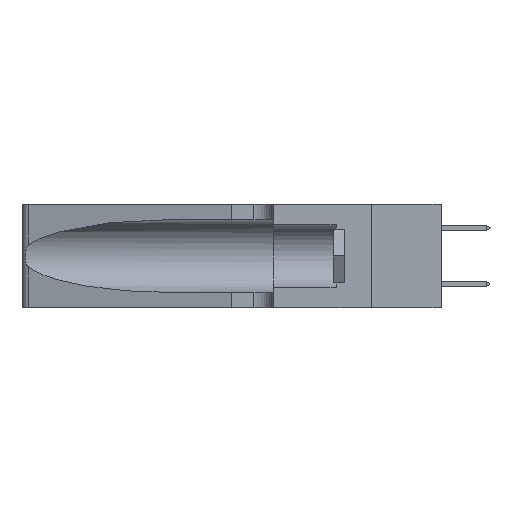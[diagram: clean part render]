
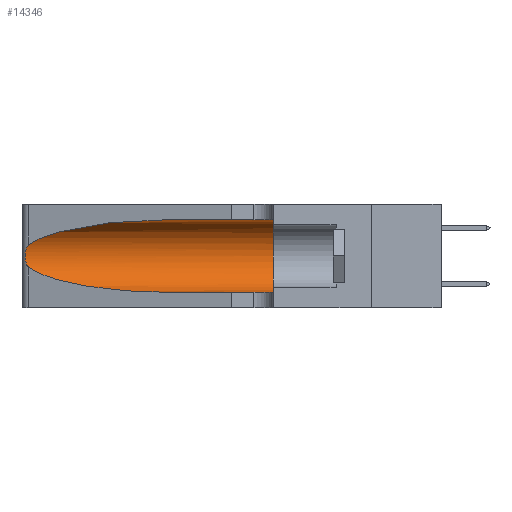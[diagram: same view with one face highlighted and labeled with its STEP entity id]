
A CAD part, left-side view. The second image highlights one B-rep face of the part: STEP entity #14346.
In plain terms, the highlighted cylindrical face has radius 3.308 mm (diameter 6.617 mm), a partial arc.
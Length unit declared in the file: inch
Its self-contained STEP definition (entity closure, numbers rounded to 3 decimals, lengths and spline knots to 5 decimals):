
#706 = DIRECTION ( 'NONE',  ( 0., -1., 0. ) ) ;
#932 = VERTEX_POINT ( 'NONE', #3091 ) ;
#1128 = CARTESIAN_POINT ( 'NONE',  ( 0.2373, 1.15595, 0.28018 ) ) ;
#1200 = CARTESIAN_POINT ( 'NONE',  ( 0.25487, 1.22718, 0.22369 ) ) ;
#1931 = VERTEX_POINT ( 'NONE', #32887 ) ;
#2377 = CARTESIAN_POINT ( 'NONE',  ( 0.2373, 1.15595, 0.08982 ) ) ;
#2533 = CARTESIAN_POINT ( 'NONE',  ( 0.26075, 1.23896, 0.19203 ) ) ;
#2657 = EDGE_CURVE ( 'NONE', #2901, #16434, #25597, .T. ) ;
#2893 = EDGE_CURVE ( 'NONE', #16434, #1931, #18274, .T. ) ;
#2901 = VERTEX_POINT ( 'NONE', #37509 ) ;
#3091 = CARTESIAN_POINT ( 'NONE',  ( 0.1305, 0.72297, 0.05475 ) ) ;
#3627 = ORIENTED_EDGE ( 'NONE', *, *, #18187, .F. ) ;
#3734 = AXIS2_PLACEMENT_3D ( 'NONE', #3744, #25972, #6998 ) ;
#3744 = CARTESIAN_POINT ( 'NONE',  ( 0.1305, 0.35, 0.185 ) ) ;
#4104 = ORIENTED_EDGE ( 'NONE', *, *, #6534, .F. ) ;
#4507 = CARTESIAN_POINT ( 'NONE',  ( 0.18966, 0.96281, 0.31525 ) ) ;
#4724 =( BOUNDED_CURVE ( )  B_SPLINE_CURVE ( 3, ( #40383, #2377, #24632, #5607 ),
 .UNSPECIFIED., .F., .F. ) 
 B_SPLINE_CURVE_WITH_KNOTS ( ( 4, 4 ),
 ( 3.44316, 4.71239 ),
 .UNSPECIFIED. ) 
 CURVE ( )  GEOMETRIC_REPRESENTATION_ITEM ( )  RATIONAL_B_SPLINE_CURVE ( ( 1., 0.87, 0.87, 1. ) ) 
 REPRESENTATION_ITEM ( '' )  );
#5063 = CARTESIAN_POINT ( 'NONE',  ( 0.1305, 0.35, 0.31525 ) ) ;
#5595 = DIRECTION ( 'NONE',  ( 0., -1., 0. ) ) ;
#5607 = CARTESIAN_POINT ( 'NONE',  ( 0.1305, 0.72297, 0.05475 ) ) ;
#5761 = CARTESIAN_POINT ( 'NONE',  ( 0.26017, 1.23833, 0.17102 ) ) ;
#6534 = EDGE_CURVE ( 'NONE', #2901, #16122, #35274, .T. ) ;
#6998 = DIRECTION ( 'NONE',  ( 0., 0., 1. ) ) ;
#8979 = CARTESIAN_POINT ( 'NONE',  ( 0.25789, 1.23486, 0.15765 ) ) ;
#9538 = DIRECTION ( 'NONE',  ( 0., 0., -1. ) ) ;
#10998 = CARTESIAN_POINT ( 'NONE',  ( 0.25487, 1.22718, 0.22369 ) ) ;
#12193 = CARTESIAN_POINT ( 'NONE',  ( 0.25555, 1.22993, 0.14849 ) ) ;
#12730 = CIRCLE ( 'NONE', #3734, 0.13025 ) ;
#14346 = ADVANCED_FACE ( 'NONE', ( #20648 ), #33510, .F. ) ;
#16107 = ORIENTED_EDGE ( 'NONE', *, *, #30903, .T. ) ;
#16122 = VERTEX_POINT ( 'NONE', #5063 ) ;
#16434 = VERTEX_POINT ( 'NONE', #1200 ) ;
#18187 = EDGE_CURVE ( 'NONE', #16122, #24683, #12730, .T. ) ;
#18274 = B_SPLINE_CURVE_WITH_KNOTS ( 'NONE', 3,
 ( #18295, #31002, #37370, #18429, #40533, #21575, #2533, #24783, #5761, #27948, #8979, #31133, #12193, #34324 ),
 .UNSPECIFIED., .F., .F.,
 ( 4, 2, 2, 2, 2, 2, 4 ),
 ( 0., 0.00027, 0.00053, 0.00107, 0.0016, 0.00187, 0.00214 ),
 .UNSPECIFIED. ) ;
#18295 = CARTESIAN_POINT ( 'NONE',  ( 0.25487, 1.22718, 0.22369 ) ) ;
#18429 = CARTESIAN_POINT ( 'NONE',  ( 0.25787, 1.23484, 0.2124 ) ) ;
#20053 = EDGE_CURVE ( 'NONE', #932, #24683, #27425, .T. ) ;
#20648 = FACE_OUTER_BOUND ( 'NONE', #21431, .T. ) ;
#21379 = ORIENTED_EDGE ( 'NONE', *, *, #2657, .T. ) ;
#21431 = EDGE_LOOP ( 'NONE', ( #21379, #26727, #16107, #35734, #3627, #4104 ) ) ;
#21575 = CARTESIAN_POINT ( 'NONE',  ( 0.26018, 1.23835, 0.19895 ) ) ;
#22123 = CARTESIAN_POINT ( 'NONE',  ( 0.1305, 1.61858, 0.185 ) ) ;
#24632 = CARTESIAN_POINT ( 'NONE',  ( 0.18966, 0.96281, 0.05475 ) ) ;
#24683 = VERTEX_POINT ( 'NONE', #31760 ) ;
#24783 = CARTESIAN_POINT ( 'NONE',  ( 0.26075, 1.23896, 0.178 ) ) ;
#25597 =( BOUNDED_CURVE ( )  B_SPLINE_CURVE ( 3, ( #29935, #4507, #1128, #10998 ),
 .UNSPECIFIED., .F., .F. ) 
 B_SPLINE_CURVE_WITH_KNOTS ( ( 4, 4 ),
 ( 1.5708, 2.84003 ),
 .UNSPECIFIED. ) 
 CURVE ( )  GEOMETRIC_REPRESENTATION_ITEM ( )  RATIONAL_B_SPLINE_CURVE ( ( 1., 0.87, 0.87, 1. ) ) 
 REPRESENTATION_ITEM ( '' )  );
#25972 = DIRECTION ( 'NONE',  ( 0., 1., 0. ) ) ;
#26727 = ORIENTED_EDGE ( 'NONE', *, *, #2893, .T. ) ;
#26852 = VECTOR ( 'NONE', #5595, 39.37008 ) ;
#27425 = LINE ( 'NONE', #29378, #28434 ) ;
#27855 = AXIS2_PLACEMENT_3D ( 'NONE', #22123, #37908, #9538 ) ;
#27948 = CARTESIAN_POINT ( 'NONE',  ( 0.25856, 1.23593, 0.16098 ) ) ;
#28434 = VECTOR ( 'NONE', #706, 39.37008 ) ;
#29378 = CARTESIAN_POINT ( 'NONE',  ( 0.1305, 1.61858, 0.05475 ) ) ;
#29935 = CARTESIAN_POINT ( 'NONE',  ( 0.1305, 0.72297, 0.31525 ) ) ;
#30848 = CARTESIAN_POINT ( 'NONE',  ( 0.1305, 1.61858, 0.31525 ) ) ;
#30903 = EDGE_CURVE ( 'NONE', #1931, #932, #4724, .T. ) ;
#31002 = CARTESIAN_POINT ( 'NONE',  ( 0.25555, 1.22994, 0.2215 ) ) ;
#31133 = CARTESIAN_POINT ( 'NONE',  ( 0.25639, 1.23186, 0.15144 ) ) ;
#31760 = CARTESIAN_POINT ( 'NONE',  ( 0.1305, 0.35, 0.05475 ) ) ;
#32887 = CARTESIAN_POINT ( 'NONE',  ( 0.25487, 1.22718, 0.14631 ) ) ;
#33510 = CYLINDRICAL_SURFACE ( 'NONE', #27855, 0.13025 ) ;
#34324 = CARTESIAN_POINT ( 'NONE',  ( 0.25487, 1.22718, 0.14631 ) ) ;
#35274 = LINE ( 'NONE', #30848, #26852 ) ;
#35734 = ORIENTED_EDGE ( 'NONE', *, *, #20053, .T. ) ;
#37370 = CARTESIAN_POINT ( 'NONE',  ( 0.25639, 1.23184, 0.21858 ) ) ;
#37509 = CARTESIAN_POINT ( 'NONE',  ( 0.1305, 0.72297, 0.31525 ) ) ;
#37908 = DIRECTION ( 'NONE',  ( 0., -1., 0. ) ) ;
#40383 = CARTESIAN_POINT ( 'NONE',  ( 0.25487, 1.22718, 0.14631 ) ) ;
#40533 = CARTESIAN_POINT ( 'NONE',  ( 0.25854, 1.2359, 0.20912 ) ) ;
